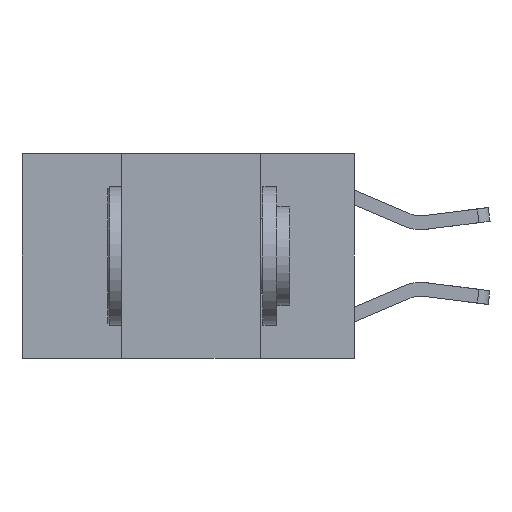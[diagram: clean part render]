
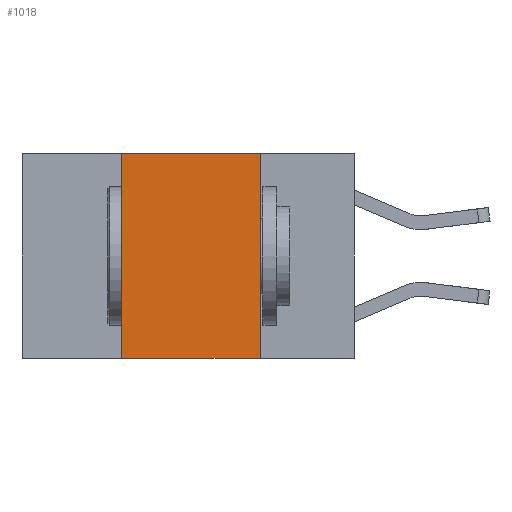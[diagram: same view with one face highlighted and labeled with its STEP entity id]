
A CAD part, left-side view. The second image highlights one B-rep face of the part: STEP entity #1018.
In plain terms, the highlighted planar face has unit normal (-1, 0, 0).
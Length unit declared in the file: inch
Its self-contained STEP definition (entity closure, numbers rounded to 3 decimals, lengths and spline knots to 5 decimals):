
#101 = CARTESIAN_POINT ( 'NONE',  ( 0., 0.42, 0. ) ) ;
#356 = VERTEX_POINT ( 'NONE', #4675 ) ;
#398 = CARTESIAN_POINT ( 'NONE',  ( 0., 0.6, 0. ) ) ;
#1018 = ADVANCED_FACE ( 'NONE', ( #3089 ), #10099, .F. ) ;
#1307 = CARTESIAN_POINT ( 'NONE',  ( 0., 0.42, -0.37 ) ) ;
#1346 = DIRECTION ( 'NONE',  ( 0., -1., 0. ) ) ;
#1438 = VERTEX_POINT ( 'NONE', #1307 ) ;
#1640 = VECTOR ( 'NONE', #5981, 39.37008 ) ;
#1664 = ORIENTED_EDGE ( 'NONE', *, *, #4454, .F. ) ;
#1865 = ORIENTED_EDGE ( 'NONE', *, *, #8375, .F. ) ;
#2882 = ORIENTED_EDGE ( 'NONE', *, *, #9337, .F. ) ;
#3035 = AXIS2_PLACEMENT_3D ( 'NONE', #398, #9609, #9584 ) ;
#3089 = FACE_OUTER_BOUND ( 'NONE', #4166, .T. ) ;
#3521 = CARTESIAN_POINT ( 'NONE',  ( 0., 0.17, -0.37 ) ) ;
#4166 = EDGE_LOOP ( 'NONE', ( #2882, #1664, #1865, #7968 ) ) ;
#4212 = CARTESIAN_POINT ( 'NONE',  ( 0., 0.42, 0. ) ) ;
#4243 = DIRECTION ( 'NONE',  ( 0., 0., 1. ) ) ;
#4454 = EDGE_CURVE ( 'NONE', #6009, #356, #10396, .T. ) ;
#4675 = CARTESIAN_POINT ( 'NONE',  ( 0., 0.17, 0. ) ) ;
#5981 = DIRECTION ( 'NONE',  ( 0., -1., 0. ) ) ;
#6009 = VERTEX_POINT ( 'NONE', #101 ) ;
#6313 = LINE ( 'NONE', #6542, #8183 ) ;
#6542 = CARTESIAN_POINT ( 'NONE',  ( 0., 0.17, 0. ) ) ;
#6823 = LINE ( 'NONE', #4212, #8710 ) ;
#7968 = ORIENTED_EDGE ( 'NONE', *, *, #8449, .T. ) ;
#8183 = VECTOR ( 'NONE', #10395, 39.37008 ) ;
#8196 = LINE ( 'NONE', #8435, #1640 ) ;
#8375 = EDGE_CURVE ( 'NONE', #1438, #6009, #6823, .T. ) ;
#8430 = VECTOR ( 'NONE', #1346, 39.37008 ) ;
#8435 = CARTESIAN_POINT ( 'NONE',  ( 0., 0.6, -0.37 ) ) ;
#8449 = EDGE_CURVE ( 'NONE', #1438, #9683, #8196, .T. ) ;
#8710 = VECTOR ( 'NONE', #4243, 39.37008 ) ;
#9337 = EDGE_CURVE ( 'NONE', #356, #9683, #6313, .T. ) ;
#9584 = DIRECTION ( 'NONE',  ( 0., 0., -1. ) ) ;
#9609 = DIRECTION ( 'NONE',  ( 1., 0., 0. ) ) ;
#9683 = VERTEX_POINT ( 'NONE', #3521 ) ;
#9723 = CARTESIAN_POINT ( 'NONE',  ( 0., 0.6, 0. ) ) ;
#10099 = PLANE ( 'NONE',  #3035 ) ;
#10395 = DIRECTION ( 'NONE',  ( 0., 0., -1. ) ) ;
#10396 = LINE ( 'NONE', #9723, #8430 ) ;
